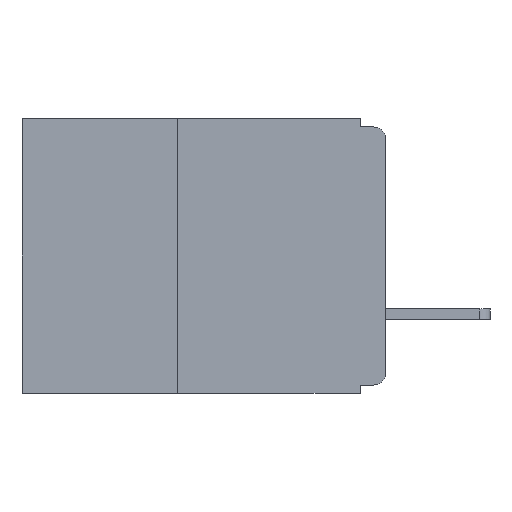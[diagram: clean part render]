
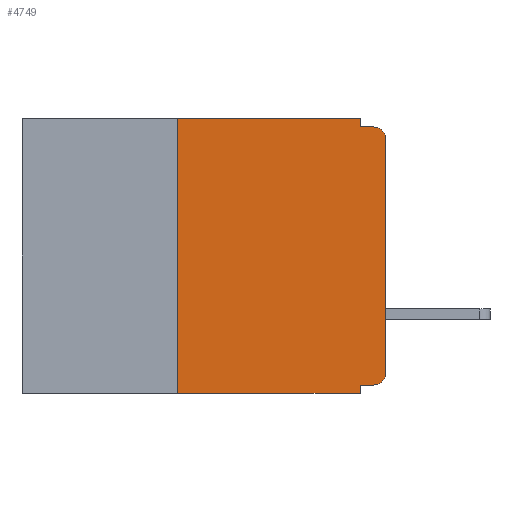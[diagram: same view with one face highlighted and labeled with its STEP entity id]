
A CAD part, left-side view. The second image highlights one B-rep face of the part: STEP entity #4749.
In plain terms, the highlighted planar face has unit normal (-1, 0, 0).
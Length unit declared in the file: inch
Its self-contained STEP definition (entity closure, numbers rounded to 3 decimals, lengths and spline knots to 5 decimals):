
#230 = LINE ( 'NONE', #2315, #15923 ) ;
#341 = CARTESIAN_POINT ( 'NONE',  ( 0., 0.25, 0. ) ) ;
#1217 = ORIENTED_EDGE ( 'NONE', *, *, #11772, .F. ) ;
#1344 = LINE ( 'NONE', #4692, #16415 ) ;
#1371 = DIRECTION ( 'NONE',  ( -1., 0., 0. ) ) ;
#1378 = VERTEX_POINT ( 'NONE', #16817 ) ;
#1948 = CARTESIAN_POINT ( 'NONE',  ( 0., 0., 0. ) ) ;
#2315 = CARTESIAN_POINT ( 'NONE',  ( 0., 0.25, -0.33 ) ) ;
#2417 = EDGE_CURVE ( 'NONE', #7031, #21510, #230, .T. ) ;
#2566 = CARTESIAN_POINT ( 'NONE',  ( 0., 0.437, 0. ) ) ;
#2657 = DIRECTION ( 'NONE',  ( 0., 1., 0. ) ) ;
#2759 = ORIENTED_EDGE ( 'NONE', *, *, #2417, .F. ) ;
#2968 = CIRCLE ( 'NONE', #22847, 0.015 ) ;
#3724 = CARTESIAN_POINT ( 'NONE',  ( 0., 0.031, 0. ) ) ;
#3738 = DIRECTION ( 'NONE',  ( -1., 0., 0. ) ) ;
#4215 = CARTESIAN_POINT ( 'NONE',  ( 0., 0.015, -0.01 ) ) ;
#4692 = CARTESIAN_POINT ( 'NONE',  ( 0., 0., -0.32 ) ) ;
#4749 = ADVANCED_FACE ( 'NONE', ( #14154 ), #9727, .F. ) ;
#5299 = CARTESIAN_POINT ( 'NONE',  ( 0., 0.031, -0.33 ) ) ;
#5476 = CARTESIAN_POINT ( 'NONE',  ( 0., 0., -0.305 ) ) ;
#5870 = EDGE_CURVE ( 'NONE', #19920, #11978, #12822, .T. ) ;
#5945 = DIRECTION ( 'NONE',  ( 0., -1., 0. ) ) ;
#6135 = VECTOR ( 'NONE', #12830, 39.37008 ) ;
#6962 = VECTOR ( 'NONE', #22561, 39.37008 ) ;
#6997 = AXIS2_PLACEMENT_3D ( 'NONE', #13771, #11795, #26268 ) ;
#7031 = VERTEX_POINT ( 'NONE', #12672 ) ;
#7218 = CARTESIAN_POINT ( 'NONE',  ( 0., 0.437, -0.33 ) ) ;
#7438 = ORIENTED_EDGE ( 'NONE', *, *, #9602, .F. ) ;
#8100 = ORIENTED_EDGE ( 'NONE', *, *, #11509, .T. ) ;
#8528 = VERTEX_POINT ( 'NONE', #15757 ) ;
#9018 = ORIENTED_EDGE ( 'NONE', *, *, #23911, .T. ) ;
#9249 = DIRECTION ( 'NONE',  ( 0., -1., 0. ) ) ;
#9397 = CARTESIAN_POINT ( 'NONE',  ( 0., 0.031, -0.33 ) ) ;
#9602 = EDGE_CURVE ( 'NONE', #23995, #24177, #12986, .T. ) ;
#9727 = PLANE ( 'NONE',  #6997 ) ;
#11295 = VERTEX_POINT ( 'NONE', #3724 ) ;
#11509 = EDGE_CURVE ( 'NONE', #1378, #24177, #2968, .T. ) ;
#11772 = EDGE_CURVE ( 'NONE', #21510, #11295, #12853, .T. ) ;
#11790 = EDGE_CURVE ( 'NONE', #8528, #19920, #1344, .T. ) ;
#11795 = DIRECTION ( 'NONE',  ( 1., 0., 0. ) ) ;
#11894 = ORIENTED_EDGE ( 'NONE', *, *, #11790, .F. ) ;
#11978 = VERTEX_POINT ( 'NONE', #5299 ) ;
#12672 = CARTESIAN_POINT ( 'NONE',  ( 0., 0.25, -0.33 ) ) ;
#12822 = LINE ( 'NONE', #9397, #18316 ) ;
#12830 = DIRECTION ( 'NONE',  ( 0., -1., 0. ) ) ;
#12853 = LINE ( 'NONE', #2566, #6135 ) ;
#12986 = LINE ( 'NONE', #22450, #22727 ) ;
#13610 = CARTESIAN_POINT ( 'NONE',  ( 0., 0.015, -0.305 ) ) ;
#13771 = CARTESIAN_POINT ( 'NONE',  ( 0., 0.437, 0. ) ) ;
#13891 = CARTESIAN_POINT ( 'NONE',  ( 0., 0.031, -0.01 ) ) ;
#13991 = LINE ( 'NONE', #7218, #23740 ) ;
#14154 = FACE_OUTER_BOUND ( 'NONE', #15178, .T. ) ;
#14725 = EDGE_CURVE ( 'NONE', #15194, #1378, #24077, .T. ) ;
#15092 = VECTOR ( 'NONE', #21415, 39.37008 ) ;
#15178 = EDGE_LOOP ( 'NONE', ( #23941, #8100, #7438, #21825, #1217, #2759, #22325, #17524, #11894, #9018 ) ) ;
#15194 = VERTEX_POINT ( 'NONE', #5476 ) ;
#15706 = DIRECTION ( 'NONE',  ( 0., 0., -1. ) ) ;
#15757 = CARTESIAN_POINT ( 'NONE',  ( 0., 0.015, -0.32 ) ) ;
#15923 = VECTOR ( 'NONE', #20168, 39.37008 ) ;
#16022 = CARTESIAN_POINT ( 'NONE',  ( 0., 0.015, -0.025 ) ) ;
#16358 = EDGE_CURVE ( 'NONE', #7031, #11978, #13991, .T. ) ;
#16374 = CARTESIAN_POINT ( 'NONE',  ( 0., 0.031, -0.32 ) ) ;
#16415 = VECTOR ( 'NONE', #2657, 39.37008 ) ;
#16817 = CARTESIAN_POINT ( 'NONE',  ( 0., 0., -0.025 ) ) ;
#17229 = CARTESIAN_POINT ( 'NONE',  ( 0., 0.031, 0. ) ) ;
#17524 = ORIENTED_EDGE ( 'NONE', *, *, #5870, .F. ) ;
#18080 = DIRECTION ( 'NONE',  ( 0., 0., -1. ) ) ;
#18316 = VECTOR ( 'NONE', #25844, 39.37008 ) ;
#19920 = VERTEX_POINT ( 'NONE', #16374 ) ;
#20168 = DIRECTION ( 'NONE',  ( 0., 0., 1. ) ) ;
#20388 = EDGE_CURVE ( 'NONE', #11295, #23995, #21239, .T. ) ;
#20475 = CIRCLE ( 'NONE', #21207, 0.015 ) ;
#21207 = AXIS2_PLACEMENT_3D ( 'NONE', #13610, #1371, #15706 ) ;
#21239 = LINE ( 'NONE', #17229, #15092 ) ;
#21415 = DIRECTION ( 'NONE',  ( 0., 0., -1. ) ) ;
#21510 = VERTEX_POINT ( 'NONE', #341 ) ;
#21825 = ORIENTED_EDGE ( 'NONE', *, *, #20388, .F. ) ;
#22325 = ORIENTED_EDGE ( 'NONE', *, *, #16358, .T. ) ;
#22450 = CARTESIAN_POINT ( 'NONE',  ( 0., 0., -0.01 ) ) ;
#22561 = DIRECTION ( 'NONE',  ( 0., 0., 1. ) ) ;
#22727 = VECTOR ( 'NONE', #5945, 39.37008 ) ;
#22847 = AXIS2_PLACEMENT_3D ( 'NONE', #16022, #3738, #18080 ) ;
#23740 = VECTOR ( 'NONE', #9249, 39.37008 ) ;
#23911 = EDGE_CURVE ( 'NONE', #8528, #15194, #20475, .T. ) ;
#23941 = ORIENTED_EDGE ( 'NONE', *, *, #14725, .T. ) ;
#23995 = VERTEX_POINT ( 'NONE', #13891 ) ;
#24077 = LINE ( 'NONE', #1948, #6962 ) ;
#24177 = VERTEX_POINT ( 'NONE', #4215 ) ;
#25844 = DIRECTION ( 'NONE',  ( 0., 0., -1. ) ) ;
#26268 = DIRECTION ( 'NONE',  ( 0., 0., -1. ) ) ;
